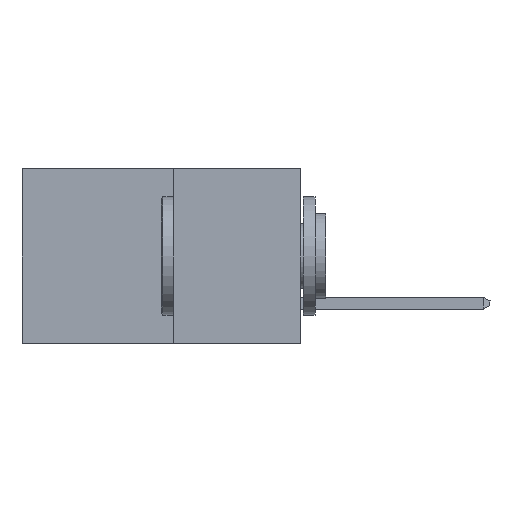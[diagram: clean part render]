
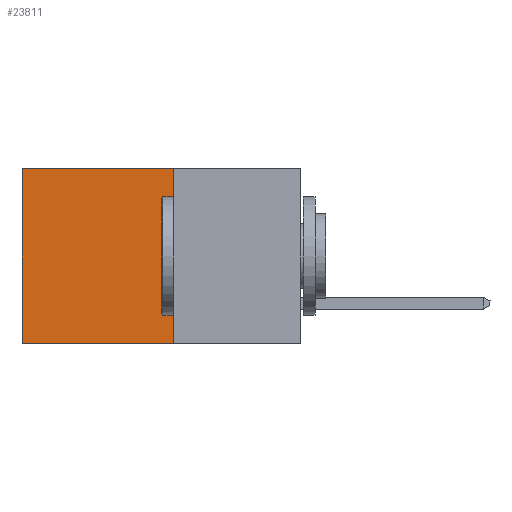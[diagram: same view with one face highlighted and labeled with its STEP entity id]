
A CAD part, left-side view. The second image highlights one B-rep face of the part: STEP entity #23811.
In plain terms, the highlighted planar face has unit normal (-1, 0, 0).
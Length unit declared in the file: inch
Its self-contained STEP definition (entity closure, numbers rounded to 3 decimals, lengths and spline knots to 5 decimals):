
#793 = ORIENTED_EDGE ( 'NONE', *, *, #24049, .T. ) ;
#2876 = CARTESIAN_POINT ( 'NONE',  ( 0.277, 0.27, -0.37 ) ) ;
#3609 = VECTOR ( 'NONE', #15612, 39.37008 ) ;
#3658 = DIRECTION ( 'NONE',  ( 0., 1., 0. ) ) ;
#3812 = EDGE_CURVE ( 'NONE', #8682, #28699, #7923, .T. ) ;
#4583 = CARTESIAN_POINT ( 'NONE',  ( 0.277, 0.59, -0.37 ) ) ;
#5006 = LINE ( 'NONE', #24482, #3609 ) ;
#5124 = DIRECTION ( 'NONE',  ( 1., 0., 0. ) ) ;
#5206 = VECTOR ( 'NONE', #3658, 39.37008 ) ;
#7923 = LINE ( 'NONE', #11561, #19233 ) ;
#8682 = VERTEX_POINT ( 'NONE', #27434 ) ;
#9250 = DIRECTION ( 'NONE',  ( 0., 1., 0. ) ) ;
#11334 = LINE ( 'NONE', #21650, #5206 ) ;
#11561 = CARTESIAN_POINT ( 'NONE',  ( 0.277, 0.27, 0. ) ) ;
#13165 = CARTESIAN_POINT ( 'NONE',  ( 0.277, 0.59, -0.37 ) ) ;
#13817 = CARTESIAN_POINT ( 'NONE',  ( 0.277, 0.27, -0.37 ) ) ;
#15375 = EDGE_LOOP ( 'NONE', ( #793, #18890, #25121, #25925 ) ) ;
#15612 = DIRECTION ( 'NONE',  ( 0., 0., -1. ) ) ;
#15898 = LINE ( 'NONE', #13165, #28489 ) ;
#16434 = PLANE ( 'NONE',  #24994 ) ;
#18890 = ORIENTED_EDGE ( 'NONE', *, *, #24620, .F. ) ;
#19233 = VECTOR ( 'NONE', #9250, 39.37008 ) ;
#19269 = EDGE_CURVE ( 'NONE', #8682, #20111, #5006, .T. ) ;
#20111 = VERTEX_POINT ( 'NONE', #13817 ) ;
#20976 = DIRECTION ( 'NONE',  ( 0., 0., -1. ) ) ;
#21650 = CARTESIAN_POINT ( 'NONE',  ( 0.277, 0.27, -0.37 ) ) ;
#23024 = VERTEX_POINT ( 'NONE', #4583 ) ;
#23811 = ADVANCED_FACE ( 'NONE', ( #27428 ), #16434, .F. ) ;
#24049 = EDGE_CURVE ( 'NONE', #28699, #23024, #15898, .T. ) ;
#24482 = CARTESIAN_POINT ( 'NONE',  ( 0.277, 0.27, -0.37 ) ) ;
#24620 = EDGE_CURVE ( 'NONE', #20111, #23024, #11334, .T. ) ;
#24994 = AXIS2_PLACEMENT_3D ( 'NONE', #2876, #5124, #20976 ) ;
#25121 = ORIENTED_EDGE ( 'NONE', *, *, #19269, .F. ) ;
#25925 = ORIENTED_EDGE ( 'NONE', *, *, #3812, .T. ) ;
#26327 = CARTESIAN_POINT ( 'NONE',  ( 0.277, 0.59, 0. ) ) ;
#26515 = DIRECTION ( 'NONE',  ( 0., 0., -1. ) ) ;
#27428 = FACE_OUTER_BOUND ( 'NONE', #15375, .T. ) ;
#27434 = CARTESIAN_POINT ( 'NONE',  ( 0.277, 0.27, 0. ) ) ;
#28489 = VECTOR ( 'NONE', #26515, 39.37008 ) ;
#28699 = VERTEX_POINT ( 'NONE', #26327 ) ;
